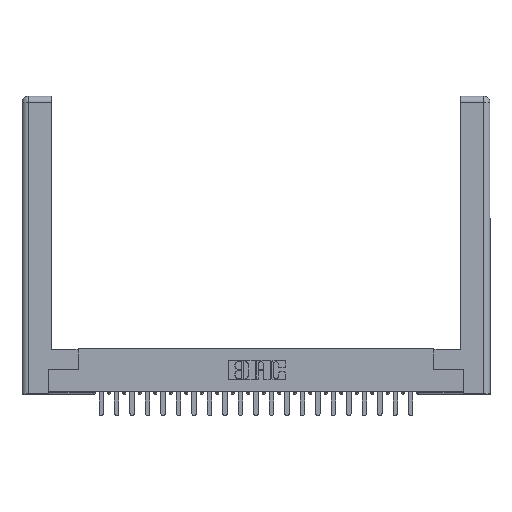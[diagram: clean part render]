
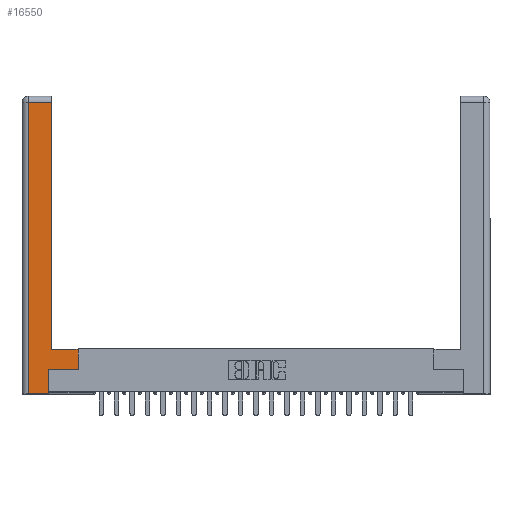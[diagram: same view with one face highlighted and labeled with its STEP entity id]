
A CAD part, top view. The second image highlights one B-rep face of the part: STEP entity #16550.
In plain terms, the highlighted planar face has unit normal (0, 0, 1).
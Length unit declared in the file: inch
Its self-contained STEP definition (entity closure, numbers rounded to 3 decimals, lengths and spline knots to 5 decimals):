
#262 = VERTEX_POINT ( 'NONE', #20904 ) ;
#1734 = VECTOR ( 'NONE', #13618, 39.37008 ) ;
#2438 = ORIENTED_EDGE ( 'NONE', *, *, #19389, .T. ) ;
#2861 = LINE ( 'NONE', #25720, #7868 ) ;
#3261 = ORIENTED_EDGE ( 'NONE', *, *, #11358, .T. ) ;
#3401 = LINE ( 'NONE', #16444, #14883 ) ;
#4950 = CARTESIAN_POINT ( 'NONE',  ( 0.565, 0.45, 0. ) ) ;
#5082 = EDGE_CURVE ( 'NONE', #9927, #21424, #27314, .T. ) ;
#6897 = CARTESIAN_POINT ( 'NONE',  ( 0.265, 0., 0. ) ) ;
#7372 = VECTOR ( 'NONE', #17544, 39.37008 ) ;
#7468 = ORIENTED_EDGE ( 'NONE', *, *, #18834, .T. ) ;
#7868 = VECTOR ( 'NONE', #10953, 39.37008 ) ;
#7903 = ORIENTED_EDGE ( 'NONE', *, *, #18263, .T. ) ;
#8477 = VECTOR ( 'NONE', #26412, 39.37008 ) ;
#8891 = CARTESIAN_POINT ( 'NONE',  ( 0.565, 0.245, 0. ) ) ;
#9011 = ORIENTED_EDGE ( 'NONE', *, *, #10163, .T. ) ;
#9468 = VERTEX_POINT ( 'NONE', #24293 ) ;
#9643 = AXIS2_PLACEMENT_3D ( 'NONE', #14441, #18829, #20883 ) ;
#9727 = DIRECTION ( 'NONE',  ( 0., 1., 0. ) ) ;
#9927 = VERTEX_POINT ( 'NONE', #27697 ) ;
#9982 = VERTEX_POINT ( 'NONE', #16820 ) ;
#10035 = VECTOR ( 'NONE', #23839, 39.37008 ) ;
#10163 = EDGE_CURVE ( 'NONE', #9468, #22138, #21322, .T. ) ;
#10953 = DIRECTION ( 'NONE',  ( -1., 0., 0. ) ) ;
#10965 = FACE_OUTER_BOUND ( 'NONE', #24565, .T. ) ;
#10992 = CARTESIAN_POINT ( 'NONE',  ( 0.0615, 0., 0. ) ) ;
#10995 = CARTESIAN_POINT ( 'NONE',  ( 0.565, 0.45, 0. ) ) ;
#11358 = EDGE_CURVE ( 'NONE', #9982, #16558, #3401, .T. ) ;
#11545 = VECTOR ( 'NONE', #9727, 39.37008 ) ;
#12400 = PLANE ( 'NONE',  #9643 ) ;
#12810 = LINE ( 'NONE', #8891, #10035 ) ;
#13267 = DIRECTION ( 'NONE',  ( 0., 1., 0. ) ) ;
#13293 = CARTESIAN_POINT ( 'NONE',  ( 0.0615, 2.94, 0. ) ) ;
#13618 = DIRECTION ( 'NONE',  ( 1., 0., 0. ) ) ;
#14441 = CARTESIAN_POINT ( 'NONE',  ( 0., 0., 0. ) ) ;
#14883 = VECTOR ( 'NONE', #20858, 39.37008 ) ;
#15554 = CARTESIAN_POINT ( 'NONE',  ( 0.265, 0.245, 0. ) ) ;
#15807 = EDGE_CURVE ( 'NONE', #22138, #9982, #2861, .T. ) ;
#16444 = CARTESIAN_POINT ( 'NONE',  ( 0.295, 3., 0. ) ) ;
#16550 = ADVANCED_FACE ( 'NONE', ( #10965 ), #12400, .F. ) ;
#16558 = VERTEX_POINT ( 'NONE', #20786 ) ;
#16820 = CARTESIAN_POINT ( 'NONE',  ( 0.295, 0.45, 0. ) ) ;
#17544 = DIRECTION ( 'NONE',  ( 0., -1., 0. ) ) ;
#17704 = ORIENTED_EDGE ( 'NONE', *, *, #23365, .T. ) ;
#18263 = EDGE_CURVE ( 'NONE', #16558, #24458, #24585, .T. ) ;
#18829 = DIRECTION ( 'NONE',  ( 0., 0., -1. ) ) ;
#18834 = EDGE_CURVE ( 'NONE', #262, #9927, #26924, .T. ) ;
#19389 = EDGE_CURVE ( 'NONE', #24458, #262, #27601, .T. ) ;
#20786 = CARTESIAN_POINT ( 'NONE',  ( 0.295, 2.94, 0. ) ) ;
#20858 = DIRECTION ( 'NONE',  ( 0., 1., 0. ) ) ;
#20883 = DIRECTION ( 'NONE',  ( -1., 0., 0. ) ) ;
#20904 = CARTESIAN_POINT ( 'NONE',  ( 0.0615, 0., 0. ) ) ;
#21322 = LINE ( 'NONE', #10995, #24328 ) ;
#21424 = VERTEX_POINT ( 'NONE', #15554 ) ;
#22113 = CARTESIAN_POINT ( 'NONE',  ( 0.265, 0.245, 0. ) ) ;
#22138 = VERTEX_POINT ( 'NONE', #4950 ) ;
#22438 = ORIENTED_EDGE ( 'NONE', *, *, #5082, .T. ) ;
#23365 = EDGE_CURVE ( 'NONE', #21424, #9468, #12810, .T. ) ;
#23839 = DIRECTION ( 'NONE',  ( 1., 0., 0. ) ) ;
#24293 = CARTESIAN_POINT ( 'NONE',  ( 0.565, 0.245, 0. ) ) ;
#24328 = VECTOR ( 'NONE', #13267, 39.37008 ) ;
#24458 = VERTEX_POINT ( 'NONE', #24760 ) ;
#24565 = EDGE_LOOP ( 'NONE', ( #3261, #7903, #2438, #7468, #22438, #17704, #9011, #27300 ) ) ;
#24585 = LINE ( 'NONE', #13293, #8477 ) ;
#24760 = CARTESIAN_POINT ( 'NONE',  ( 0.0615, 2.94, 0. ) ) ;
#25720 = CARTESIAN_POINT ( 'NONE',  ( 0.295, 0.45, 0. ) ) ;
#26412 = DIRECTION ( 'NONE',  ( -1., 0., 0. ) ) ;
#26924 = LINE ( 'NONE', #6897, #1734 ) ;
#27300 = ORIENTED_EDGE ( 'NONE', *, *, #15807, .T. ) ;
#27314 = LINE ( 'NONE', #22113, #11545 ) ;
#27601 = LINE ( 'NONE', #10992, #7372 ) ;
#27697 = CARTESIAN_POINT ( 'NONE',  ( 0.265, 0., 0. ) ) ;
